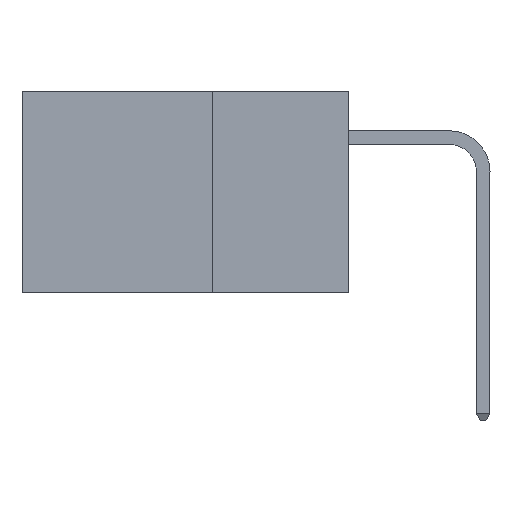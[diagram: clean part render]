
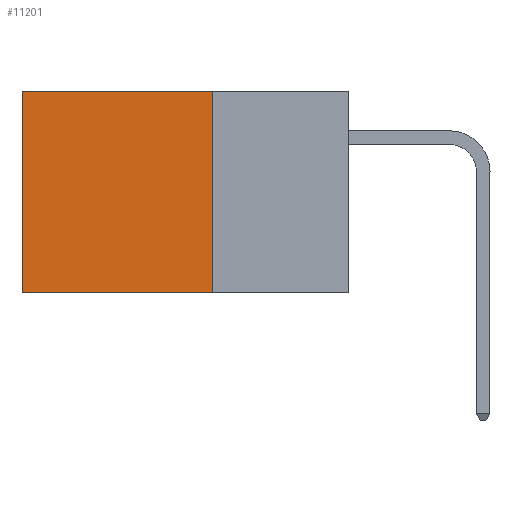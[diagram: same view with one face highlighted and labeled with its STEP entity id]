
A CAD part, left-side view. The second image highlights one B-rep face of the part: STEP entity #11201.
In plain terms, the highlighted planar face has unit normal (-1, 0, 0).
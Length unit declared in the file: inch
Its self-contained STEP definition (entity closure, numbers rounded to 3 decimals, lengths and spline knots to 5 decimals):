
#42 = AXIS2_PLACEMENT_3D ( 'NONE', #6281, #9554, #4356 ) ;
#170 = DIRECTION ( 'NONE',  ( 0., 1., 0. ) ) ;
#622 = VECTOR ( 'NONE', #6130, 39.37008 ) ;
#640 = LINE ( 'NONE', #8669, #622 ) ;
#1003 = CARTESIAN_POINT ( 'NONE',  ( 0.2875, 0.25, -0.37 ) ) ;
#1243 = VECTOR ( 'NONE', #10149, 39.37008 ) ;
#1354 = CARTESIAN_POINT ( 'NONE',  ( 0.2875, 0.25, 0. ) ) ;
#1533 = LINE ( 'NONE', #6232, #1243 ) ;
#2440 = EDGE_CURVE ( 'NONE', #9141, #4622, #2808, .T. ) ;
#2496 = CARTESIAN_POINT ( 'NONE',  ( 0.2875, 0.6, -0.37 ) ) ;
#2796 = VECTOR ( 'NONE', #3353, 39.37008 ) ;
#2808 = LINE ( 'NONE', #8850, #2796 ) ;
#2951 = CARTESIAN_POINT ( 'NONE',  ( 0.2875, 0.6, 0. ) ) ;
#3145 = VECTOR ( 'NONE', #170, 39.37008 ) ;
#3309 = LINE ( 'NONE', #7348, #3145 ) ;
#3353 = DIRECTION ( 'NONE',  ( 0., 0., -1. ) ) ;
#4356 = DIRECTION ( 'NONE',  ( 0., 0., -1. ) ) ;
#4622 = VERTEX_POINT ( 'NONE', #2496 ) ;
#5036 = EDGE_CURVE ( 'NONE', #6205, #9141, #3309, .T. ) ;
#6130 = DIRECTION ( 'NONE',  ( 0., 1., 0. ) ) ;
#6205 = VERTEX_POINT ( 'NONE', #1354 ) ;
#6232 = CARTESIAN_POINT ( 'NONE',  ( 0.2875, 0.25, 0. ) ) ;
#6281 = CARTESIAN_POINT ( 'NONE',  ( 0.2875, 0.25, 0. ) ) ;
#6587 = FACE_OUTER_BOUND ( 'NONE', #9729, .T. ) ;
#6775 = VERTEX_POINT ( 'NONE', #1003 ) ;
#7227 = ORIENTED_EDGE ( 'NONE', *, *, #2440, .T. ) ;
#7348 = CARTESIAN_POINT ( 'NONE',  ( 0.2875, 0.25, 0. ) ) ;
#7374 = ORIENTED_EDGE ( 'NONE', *, *, #10551, .F. ) ;
#7757 = ORIENTED_EDGE ( 'NONE', *, *, #8090, .F. ) ;
#8090 = EDGE_CURVE ( 'NONE', #6205, #6775, #1533, .T. ) ;
#8183 = ORIENTED_EDGE ( 'NONE', *, *, #5036, .T. ) ;
#8669 = CARTESIAN_POINT ( 'NONE',  ( 0.2875, 0.25, -0.37 ) ) ;
#8813 = PLANE ( 'NONE',  #42 ) ;
#8850 = CARTESIAN_POINT ( 'NONE',  ( 0.2875, 0.6, 0. ) ) ;
#9141 = VERTEX_POINT ( 'NONE', #2951 ) ;
#9554 = DIRECTION ( 'NONE',  ( 1., 0., 0. ) ) ;
#9729 = EDGE_LOOP ( 'NONE', ( #7227, #7374, #7757, #8183 ) ) ;
#10149 = DIRECTION ( 'NONE',  ( 0., 0., -1. ) ) ;
#10551 = EDGE_CURVE ( 'NONE', #6775, #4622, #640, .T. ) ;
#11201 = ADVANCED_FACE ( 'NONE', ( #6587 ), #8813, .F. ) ;
